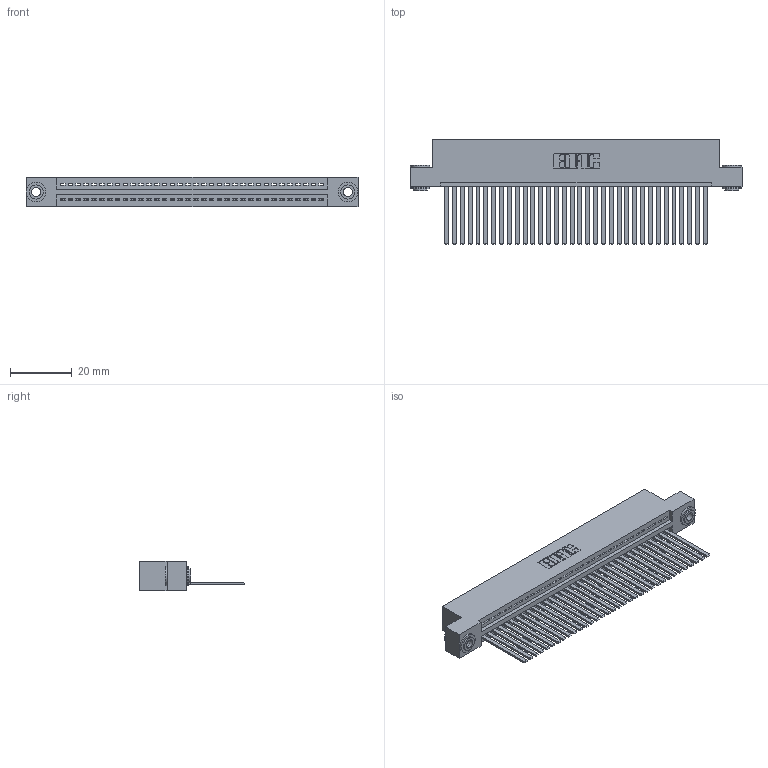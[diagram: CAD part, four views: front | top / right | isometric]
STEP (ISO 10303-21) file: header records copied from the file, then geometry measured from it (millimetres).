
FILE_DESCRIPTION (( 'STEP AP203' ), '1' );
FILE_NAME ('345-034-544-103.STEP', '2019-10-07T19:40:53', ( '' ), ( '' ), 'SwSTEP 2.0', 'SolidWorks 2016', '' );
FILE_SCHEMA (( 'CONFIG_CONTROL_DESIGN' ));
Length unit declared in the file: inch
Products named in the file (4): 345-250-002_345-250-002-102; 345-034-544-103; 345 Part_Flush Mounting Lugs - 0.156 Dia-TH; 345-292-001_345-293-144
Assembly tree (37 placements, depth 2):
  345-034-544-103
    345 Part_Flush Mounting Lugs - 0.156 Dia-TH
    345-292-001_345-293-144  x34
    345-250-002_345-250-002-102  x2
Bounding box: 107.57 x 33.96 x 9.4 mm (x, y, z)
Volume: 10564.6 mm3; surface area: 15327.3 mm2
Topology: 37 solids, 37 shells, 1932 faces, 5789 edges, 3810 vertices
Faces by surface type: plane 1314, cylinder 610, cone 8
Entity records: 27132 total; most frequent: CARTESIAN_POINT 4677, ORIENTED_EDGE 4638, DIRECTION 4125, EDGE_CURVE 2319, VECTOR 2031, LINE 2031, VERTEX_POINT 1542, AXIS2_PLACEMENT_3D 1047
